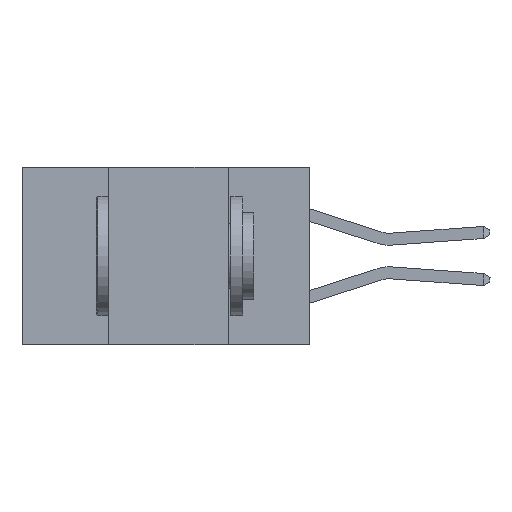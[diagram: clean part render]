
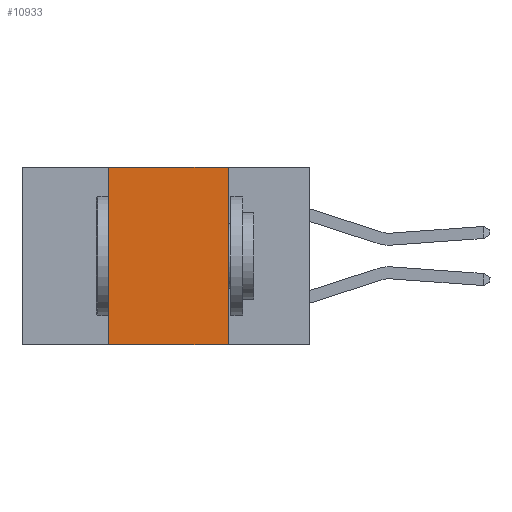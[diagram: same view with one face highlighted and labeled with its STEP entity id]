
A CAD part, left-side view. The second image highlights one B-rep face of the part: STEP entity #10933.
In plain terms, the highlighted planar face has unit normal (-1, 0, 0).
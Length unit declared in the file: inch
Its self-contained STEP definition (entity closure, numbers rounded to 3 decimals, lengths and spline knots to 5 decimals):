
#30 = CARTESIAN_POINT ( 'NONE',  ( 0., 0.6, 0. ) ) ;
#195 = CARTESIAN_POINT ( 'NONE',  ( 0., 0.42, 0. ) ) ;
#289 = CARTESIAN_POINT ( 'NONE',  ( 0., 0.42, 0. ) ) ;
#863 = VECTOR ( 'NONE', #2068, 39.37008 ) ;
#993 = DIRECTION ( 'NONE',  ( 0., -1., 0. ) ) ;
#1329 = EDGE_LOOP ( 'NONE', ( #9476, #9522, #9962, #1830 ) ) ;
#1429 = DIRECTION ( 'NONE',  ( 0., 0., 1. ) ) ;
#1643 = CARTESIAN_POINT ( 'NONE',  ( 0., 0.42, -0.37 ) ) ;
#1830 = ORIENTED_EDGE ( 'NONE', *, *, #15320, .T. ) ;
#1896 = LINE ( 'NONE', #14885, #11380 ) ;
#2064 = AXIS2_PLACEMENT_3D ( 'NONE', #30, #5077, #3896 ) ;
#2068 = DIRECTION ( 'NONE',  ( 0., -1., 0. ) ) ;
#2373 = CARTESIAN_POINT ( 'NONE',  ( 0., 0.17, -0.37 ) ) ;
#2424 = VERTEX_POINT ( 'NONE', #8744 ) ;
#3896 = DIRECTION ( 'NONE',  ( 0., 0., -1. ) ) ;
#4509 = FACE_OUTER_BOUND ( 'NONE', #1329, .T. ) ;
#4560 = CARTESIAN_POINT ( 'NONE',  ( 0., 0.6, 0. ) ) ;
#4666 = EDGE_CURVE ( 'NONE', #12170, #2424, #11559, .T. ) ;
#5077 = DIRECTION ( 'NONE',  ( 1., 0., 0. ) ) ;
#5152 = DIRECTION ( 'NONE',  ( 0., 0., -1. ) ) ;
#5627 = VERTEX_POINT ( 'NONE', #2373 ) ;
#5735 = LINE ( 'NONE', #11855, #863 ) ;
#5926 = LINE ( 'NONE', #195, #9575 ) ;
#7436 = PLANE ( 'NONE',  #2064 ) ;
#8744 = CARTESIAN_POINT ( 'NONE',  ( 0., 0.17, 0. ) ) ;
#9476 = ORIENTED_EDGE ( 'NONE', *, *, #13793, .F. ) ;
#9522 = ORIENTED_EDGE ( 'NONE', *, *, #4666, .F. ) ;
#9575 = VECTOR ( 'NONE', #1429, 39.37008 ) ;
#9962 = ORIENTED_EDGE ( 'NONE', *, *, #15025, .F. ) ;
#10712 = VERTEX_POINT ( 'NONE', #1643 ) ;
#10933 = ADVANCED_FACE ( 'NONE', ( #4509 ), #7436, .F. ) ;
#11380 = VECTOR ( 'NONE', #5152, 39.37008 ) ;
#11559 = LINE ( 'NONE', #4560, #14599 ) ;
#11855 = CARTESIAN_POINT ( 'NONE',  ( 0., 0.6, -0.37 ) ) ;
#12170 = VERTEX_POINT ( 'NONE', #289 ) ;
#13793 = EDGE_CURVE ( 'NONE', #2424, #5627, #1896, .T. ) ;
#14599 = VECTOR ( 'NONE', #993, 39.37008 ) ;
#14885 = CARTESIAN_POINT ( 'NONE',  ( 0., 0.17, 0. ) ) ;
#15025 = EDGE_CURVE ( 'NONE', #10712, #12170, #5926, .T. ) ;
#15320 = EDGE_CURVE ( 'NONE', #10712, #5627, #5735, .T. ) ;
